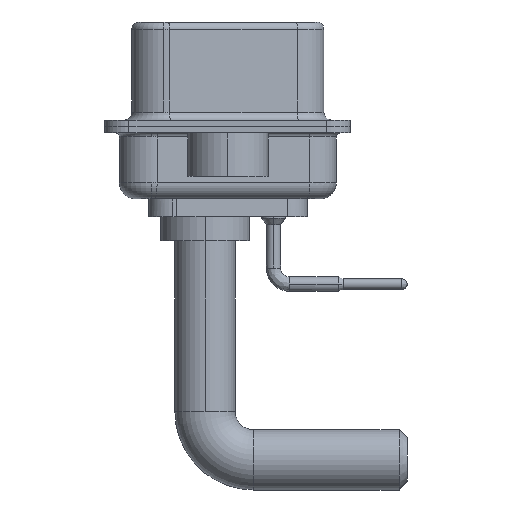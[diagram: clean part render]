
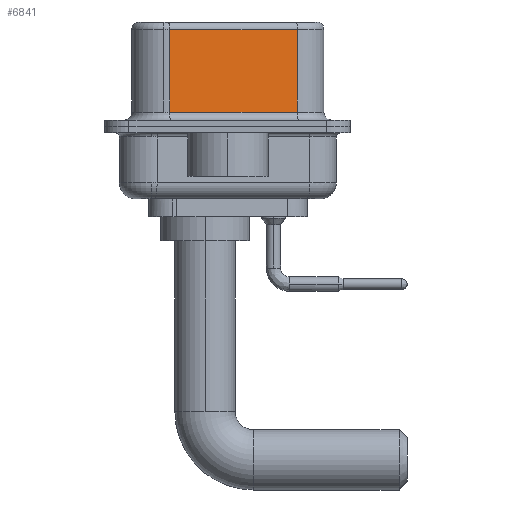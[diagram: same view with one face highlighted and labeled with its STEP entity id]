
A CAD part, left-side view. The second image highlights one B-rep face of the part: STEP entity #6841.
In plain terms, the highlighted planar face has unit normal (-0.985, -0.174, 0).
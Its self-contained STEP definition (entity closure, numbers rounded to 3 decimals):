
#867 = CARTESIAN_POINT ( 'NONE',  ( 3.73, 3.628, 6.52 ) ) ;
#931 = VERTEX_POINT ( 'NONE', #3113 ) ;
#1056 = DIRECTION ( 'NONE',  ( 0.174, -0.985, 0. ) ) ;
#1195 = DIRECTION ( 'NONE',  ( 0.985, 0.174, 0. ) ) ;
#1759 = EDGE_CURVE ( 'NONE', #5193, #23080, #8151, .T. ) ;
#2558 = DIRECTION ( 'NONE',  ( 0., 0., -1. ) ) ;
#2792 = EDGE_CURVE ( 'NONE', #931, #5193, #6515, .T. ) ;
#3012 = PLANE ( 'NONE',  #18067 ) ;
#3113 = CARTESIAN_POINT ( 'NONE',  ( 5.132, -4.322, 6.02 ) ) ;
#4524 = LINE ( 'NONE', #9968, #19395 ) ;
#5193 = VERTEX_POINT ( 'NONE', #19851 ) ;
#5628 = EDGE_CURVE ( 'NONE', #23080, #20514, #14122, .T. ) ;
#6048 = VECTOR ( 'NONE', #2558, 1000. ) ;
#6340 = CARTESIAN_POINT ( 'NONE',  ( 3.73, 3.628, 0.9 ) ) ;
#6515 = LINE ( 'NONE', #23301, #20892 ) ;
#6531 = FACE_OUTER_BOUND ( 'NONE', #15418, .T. ) ;
#6657 = CARTESIAN_POINT ( 'NONE',  ( 5.132, -4.322, 6.52 ) ) ;
#6841 = ADVANCED_FACE ( 'NONE', ( #6531 ), #3012, .F. ) ;
#8151 = LINE ( 'NONE', #867, #6048 ) ;
#9166 = VECTOR ( 'NONE', #1056, 1000. ) ;
#9663 = ORIENTED_EDGE ( 'NONE', *, *, #2792, .T. ) ;
#9968 = CARTESIAN_POINT ( 'NONE',  ( 5.132, -4.322, 6.52 ) ) ;
#11818 = DIRECTION ( 'NONE',  ( -0.174, 0.985, 0. ) ) ;
#12394 = DIRECTION ( 'NONE',  ( 0., 0., -1. ) ) ;
#12425 = ORIENTED_EDGE ( 'NONE', *, *, #1759, .T. ) ;
#13610 = CARTESIAN_POINT ( 'NONE',  ( 5.132, -4.322, 0.9 ) ) ;
#14122 = LINE ( 'NONE', #21257, #9166 ) ;
#15418 = EDGE_LOOP ( 'NONE', ( #20530, #9663, #12425, #17168 ) ) ;
#17168 = ORIENTED_EDGE ( 'NONE', *, *, #5628, .T. ) ;
#18067 = AXIS2_PLACEMENT_3D ( 'NONE', #6657, #1195, #23069 ) ;
#19395 = VECTOR ( 'NONE', #12394, 1000. ) ;
#19851 = CARTESIAN_POINT ( 'NONE',  ( 3.73, 3.628, 6.02 ) ) ;
#20514 = VERTEX_POINT ( 'NONE', #13610 ) ;
#20530 = ORIENTED_EDGE ( 'NONE', *, *, #23030, .F. ) ;
#20892 = VECTOR ( 'NONE', #11818, 1000. ) ;
#21257 = CARTESIAN_POINT ( 'NONE',  ( 5.132, -4.322, 0.9 ) ) ;
#23030 = EDGE_CURVE ( 'NONE', #931, #20514, #4524, .T. ) ;
#23069 = DIRECTION ( 'NONE',  ( -0.174, 0.985, 0. ) ) ;
#23080 = VERTEX_POINT ( 'NONE', #6340 ) ;
#23301 = CARTESIAN_POINT ( 'NONE',  ( 5.132, -4.322, 6.02 ) ) ;
